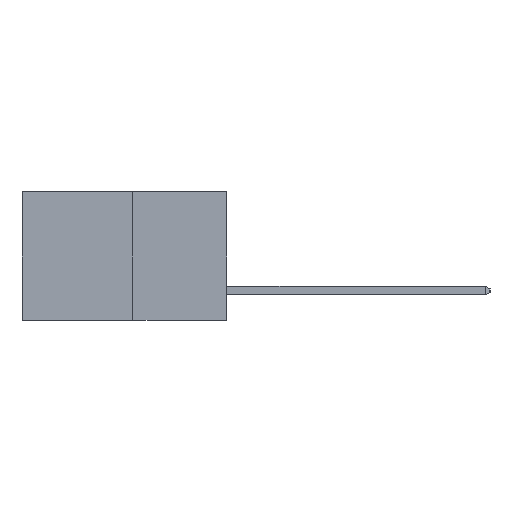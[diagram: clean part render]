
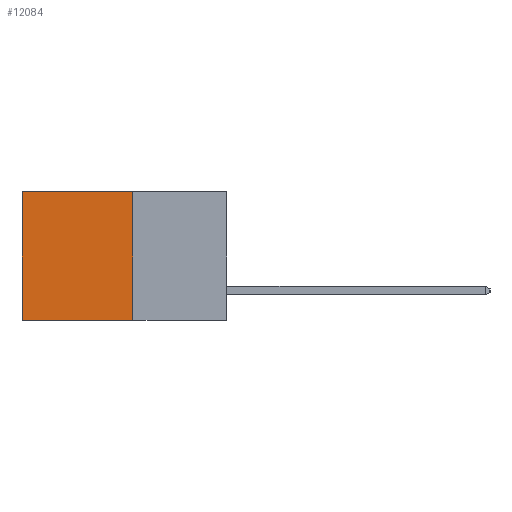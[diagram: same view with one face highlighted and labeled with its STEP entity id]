
A CAD part, left-side view. The second image highlights one B-rep face of the part: STEP entity #12084.
In plain terms, the highlighted planar face has unit normal (-1, 0, 0).
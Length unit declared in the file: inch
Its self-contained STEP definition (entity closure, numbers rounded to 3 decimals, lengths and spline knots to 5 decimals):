
#61 = EDGE_CURVE ( 'NONE', #6078, #12433, #3126, .T. ) ;
#396 = VECTOR ( 'NONE', #6060, 39.37008 ) ;
#458 = VECTOR ( 'NONE', #1503, 39.37008 ) ;
#501 = ORIENTED_EDGE ( 'NONE', *, *, #7712, .F. ) ;
#1190 = DIRECTION ( 'NONE',  ( 0., 0., -1. ) ) ;
#1408 = VERTEX_POINT ( 'NONE', #3234 ) ;
#1441 = ORIENTED_EDGE ( 'NONE', *, *, #14437, .T. ) ;
#1503 = DIRECTION ( 'NONE',  ( 0., 1., 0. ) ) ;
#1510 = CARTESIAN_POINT ( 'NONE',  ( 0.277, 0.27, -0.37 ) ) ;
#1933 = ORIENTED_EDGE ( 'NONE', *, *, #3309, .T. ) ;
#1942 = FACE_OUTER_BOUND ( 'NONE', #6508, .T. ) ;
#2314 = PLANE ( 'NONE',  #3582 ) ;
#2441 = DIRECTION ( 'NONE',  ( 0., 1., 0. ) ) ;
#3126 = LINE ( 'NONE', #1510, #8951 ) ;
#3234 = CARTESIAN_POINT ( 'NONE',  ( 0.277, 0.59, -0.37 ) ) ;
#3309 = EDGE_CURVE ( 'NONE', #6472, #1408, #9353, .T. ) ;
#3582 = AXIS2_PLACEMENT_3D ( 'NONE', #13866, #8186, #1190 ) ;
#5227 = ORIENTED_EDGE ( 'NONE', *, *, #61, .F. ) ;
#5397 = CARTESIAN_POINT ( 'NONE',  ( 0.277, 0.59, -0.37 ) ) ;
#6060 = DIRECTION ( 'NONE',  ( 0., 0., -1. ) ) ;
#6078 = VERTEX_POINT ( 'NONE', #12225 ) ;
#6251 = CARTESIAN_POINT ( 'NONE',  ( 0.277, 0.27, -0.37 ) ) ;
#6472 = VERTEX_POINT ( 'NONE', #10692 ) ;
#6508 = EDGE_LOOP ( 'NONE', ( #1933, #501, #5227, #1441 ) ) ;
#7669 = CARTESIAN_POINT ( 'NONE',  ( 0.277, 0.27, -0.37 ) ) ;
#7712 = EDGE_CURVE ( 'NONE', #12433, #1408, #9760, .T. ) ;
#8186 = DIRECTION ( 'NONE',  ( 1., 0., 0. ) ) ;
#8951 = VECTOR ( 'NONE', #9846, 39.37008 ) ;
#9353 = LINE ( 'NONE', #5397, #396 ) ;
#9760 = LINE ( 'NONE', #6251, #458 ) ;
#9846 = DIRECTION ( 'NONE',  ( 0., 0., -1. ) ) ;
#10692 = CARTESIAN_POINT ( 'NONE',  ( 0.277, 0.59, 0. ) ) ;
#11664 = CARTESIAN_POINT ( 'NONE',  ( 0.277, 0.27, 0. ) ) ;
#12084 = ADVANCED_FACE ( 'NONE', ( #1942 ), #2314, .F. ) ;
#12157 = LINE ( 'NONE', #11664, #14477 ) ;
#12225 = CARTESIAN_POINT ( 'NONE',  ( 0.277, 0.27, 0. ) ) ;
#12433 = VERTEX_POINT ( 'NONE', #7669 ) ;
#13866 = CARTESIAN_POINT ( 'NONE',  ( 0.277, 0.27, -0.37 ) ) ;
#14437 = EDGE_CURVE ( 'NONE', #6078, #6472, #12157, .T. ) ;
#14477 = VECTOR ( 'NONE', #2441, 39.37008 ) ;
